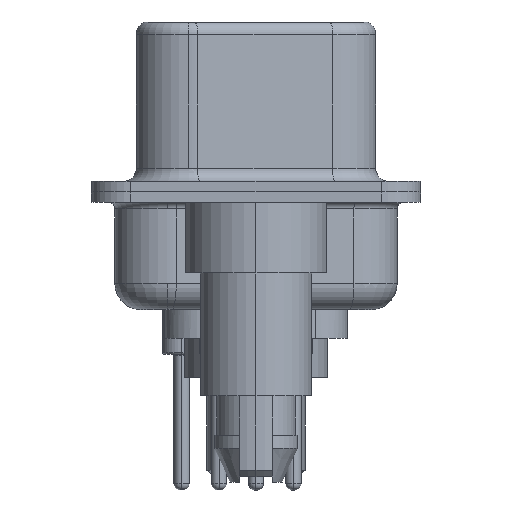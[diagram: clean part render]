
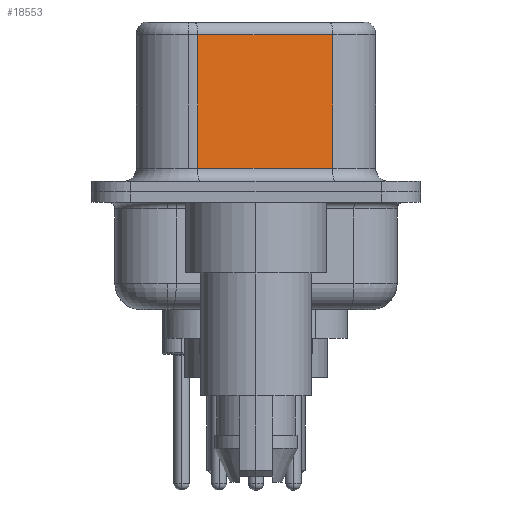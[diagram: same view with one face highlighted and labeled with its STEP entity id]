
A CAD part, left-side view. The second image highlights one B-rep face of the part: STEP entity #18553.
In plain terms, the highlighted planar face has unit normal (-0.985, -0.174, 0).
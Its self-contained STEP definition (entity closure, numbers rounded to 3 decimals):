
#307 = VERTEX_POINT ( 'NONE', #21233 ) ;
#1328 = ORIENTED_EDGE ( 'NONE', *, *, #9958, .T. ) ;
#1630 = VECTOR ( 'NONE', #18704, 1000. ) ;
#2049 = VECTOR ( 'NONE', #11087, 1000. ) ;
#2267 = AXIS2_PLACEMENT_3D ( 'NONE', #13313, #13171, #20123 ) ;
#3116 = DIRECTION ( 'NONE',  ( 0., 0., -1. ) ) ;
#4299 = EDGE_CURVE ( 'NONE', #307, #17690, #10878, .T. ) ;
#4757 = PLANE ( 'NONE',  #2267 ) ;
#4978 = LINE ( 'NONE', #17059, #1630 ) ;
#6175 = ORIENTED_EDGE ( 'NONE', *, *, #13888, .T. ) ;
#7404 = LINE ( 'NONE', #12957, #10285 ) ;
#7556 = VERTEX_POINT ( 'NONE', #13254 ) ;
#9538 = VERTEX_POINT ( 'NONE', #16419 ) ;
#9613 = VECTOR ( 'NONE', #13414, 1000. ) ;
#9958 = EDGE_CURVE ( 'NONE', #9538, #7556, #4978, .T. ) ;
#10205 = ORIENTED_EDGE ( 'NONE', *, *, #4299, .T. ) ;
#10285 = VECTOR ( 'NONE', #3116, 1000. ) ;
#10878 = LINE ( 'NONE', #21059, #2049 ) ;
#11087 = DIRECTION ( 'NONE',  ( -0.174, 0.985, 0. ) ) ;
#11216 = EDGE_CURVE ( 'NONE', #307, #7556, #14005, .T. ) ;
#12957 = CARTESIAN_POINT ( 'NONE',  ( 3.675, 2.233, 6.52 ) ) ;
#13171 = DIRECTION ( 'NONE',  ( 0.985, 0.174, 0. ) ) ;
#13254 = CARTESIAN_POINT ( 'NONE',  ( 4.585, -2.927, 0.9 ) ) ;
#13313 = CARTESIAN_POINT ( 'NONE',  ( 4.585, -2.927, 6.52 ) ) ;
#13414 = DIRECTION ( 'NONE',  ( 0., 0., -1. ) ) ;
#13888 = EDGE_CURVE ( 'NONE', #17690, #9538, #7404, .T. ) ;
#14005 = LINE ( 'NONE', #16593, #9613 ) ;
#16419 = CARTESIAN_POINT ( 'NONE',  ( 3.675, 2.233, 0.9 ) ) ;
#16593 = CARTESIAN_POINT ( 'NONE',  ( 4.585, -2.927, 6.52 ) ) ;
#17059 = CARTESIAN_POINT ( 'NONE',  ( 4.585, -2.927, 0.9 ) ) ;
#17326 = EDGE_LOOP ( 'NONE', ( #20507, #10205, #6175, #1328 ) ) ;
#17591 = CARTESIAN_POINT ( 'NONE',  ( 3.675, 2.233, 6.02 ) ) ;
#17690 = VERTEX_POINT ( 'NONE', #17591 ) ;
#18553 = ADVANCED_FACE ( 'NONE', ( #19948 ), #4757, .F. ) ;
#18704 = DIRECTION ( 'NONE',  ( 0.174, -0.985, 0. ) ) ;
#19948 = FACE_OUTER_BOUND ( 'NONE', #17326, .T. ) ;
#20123 = DIRECTION ( 'NONE',  ( -0.174, 0.985, 0. ) ) ;
#20507 = ORIENTED_EDGE ( 'NONE', *, *, #11216, .F. ) ;
#21059 = CARTESIAN_POINT ( 'NONE',  ( 4.585, -2.927, 6.02 ) ) ;
#21233 = CARTESIAN_POINT ( 'NONE',  ( 4.585, -2.927, 6.02 ) ) ;
